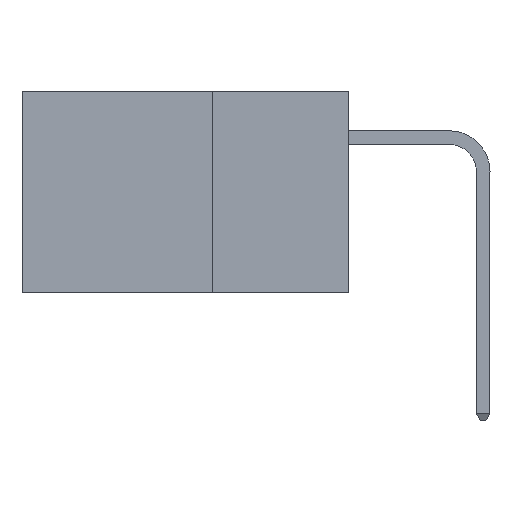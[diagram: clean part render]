
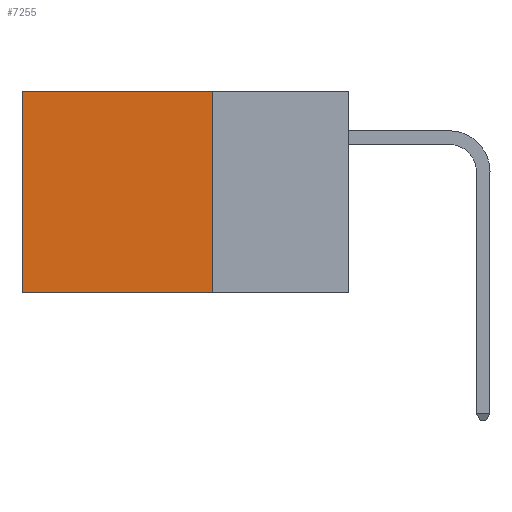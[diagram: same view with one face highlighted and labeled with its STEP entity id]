
A CAD part, left-side view. The second image highlights one B-rep face of the part: STEP entity #7255.
In plain terms, the highlighted planar face has unit normal (-1, 0, 0).
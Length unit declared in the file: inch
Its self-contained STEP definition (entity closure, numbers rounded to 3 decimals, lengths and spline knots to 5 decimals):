
#654 = CARTESIAN_POINT ( 'NONE',  ( 0.2875, 0.25, -0.37 ) ) ;
#1262 = CARTESIAN_POINT ( 'NONE',  ( 0.2875, 0.25, 0. ) ) ;
#3789 = ORIENTED_EDGE ( 'NONE', *, *, #7687, .T. ) ;
#5092 = ORIENTED_EDGE ( 'NONE', *, *, #12956, .F. ) ;
#5275 = CARTESIAN_POINT ( 'NONE',  ( 0.2875, 0.25, 0. ) ) ;
#5510 = DIRECTION ( 'NONE',  ( 0., 1., 0. ) ) ;
#6000 = EDGE_LOOP ( 'NONE', ( #3789, #22343, #5092, #21828 ) ) ;
#6498 = DIRECTION ( 'NONE',  ( 0., 0., -1. ) ) ;
#6578 = VECTOR ( 'NONE', #5510, 39.37008 ) ;
#7243 = CARTESIAN_POINT ( 'NONE',  ( 0.2875, 0.25, -0.37 ) ) ;
#7255 = ADVANCED_FACE ( 'NONE', ( #24068 ), #19756, .F. ) ;
#7687 = EDGE_CURVE ( 'NONE', #23979, #7696, #10780, .T. ) ;
#7696 = VERTEX_POINT ( 'NONE', #11257 ) ;
#8277 = EDGE_CURVE ( 'NONE', #26759, #23979, #26874, .T. ) ;
#10780 = LINE ( 'NONE', #32363, #24863 ) ;
#11257 = CARTESIAN_POINT ( 'NONE',  ( 0.2875, 0.6, -0.37 ) ) ;
#12061 = CARTESIAN_POINT ( 'NONE',  ( 0.2875, 0.6, 0. ) ) ;
#12396 = CARTESIAN_POINT ( 'NONE',  ( 0.2875, 0.25, 0. ) ) ;
#12597 = DIRECTION ( 'NONE',  ( 0., 1., 0. ) ) ;
#12956 = EDGE_CURVE ( 'NONE', #26759, #27090, #13278, .T. ) ;
#13226 = VECTOR ( 'NONE', #12597, 39.37008 ) ;
#13278 = LINE ( 'NONE', #12396, #26504 ) ;
#15078 = DIRECTION ( 'NONE',  ( 0., 0., -1. ) ) ;
#16594 = DIRECTION ( 'NONE',  ( 0., 0., -1. ) ) ;
#19756 = PLANE ( 'NONE',  #25930 ) ;
#20292 = LINE ( 'NONE', #7243, #13226 ) ;
#21828 = ORIENTED_EDGE ( 'NONE', *, *, #8277, .T. ) ;
#22343 = ORIENTED_EDGE ( 'NONE', *, *, #31309, .F. ) ;
#22395 = DIRECTION ( 'NONE',  ( 1., 0., 0. ) ) ;
#23979 = VERTEX_POINT ( 'NONE', #12061 ) ;
#24052 = CARTESIAN_POINT ( 'NONE',  ( 0.2875, 0.25, 0. ) ) ;
#24068 = FACE_OUTER_BOUND ( 'NONE', #6000, .T. ) ;
#24863 = VECTOR ( 'NONE', #16594, 39.37008 ) ;
#25930 = AXIS2_PLACEMENT_3D ( 'NONE', #1262, #22395, #6498 ) ;
#26504 = VECTOR ( 'NONE', #15078, 39.37008 ) ;
#26759 = VERTEX_POINT ( 'NONE', #5275 ) ;
#26874 = LINE ( 'NONE', #24052, #6578 ) ;
#27090 = VERTEX_POINT ( 'NONE', #654 ) ;
#31309 = EDGE_CURVE ( 'NONE', #27090, #7696, #20292, .T. ) ;
#32363 = CARTESIAN_POINT ( 'NONE',  ( 0.2875, 0.6, 0. ) ) ;
